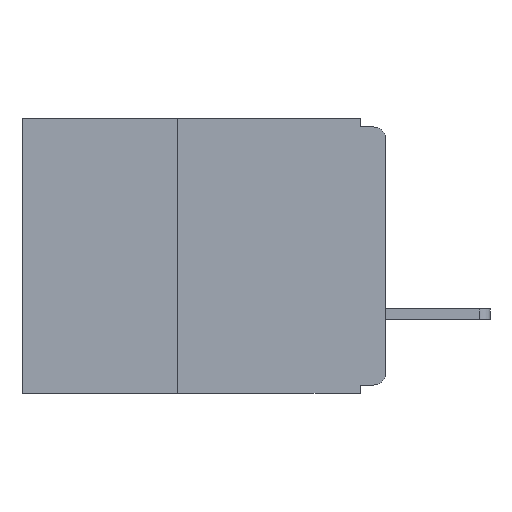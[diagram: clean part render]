
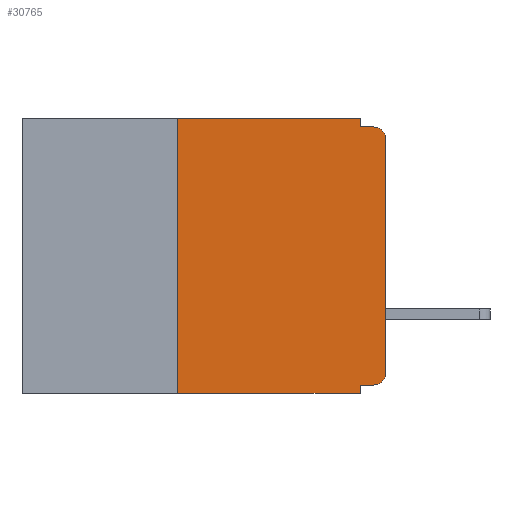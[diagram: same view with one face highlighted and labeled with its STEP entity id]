
A CAD part, left-side view. The second image highlights one B-rep face of the part: STEP entity #30765.
In plain terms, the highlighted planar face has unit normal (-1, 0, 0).
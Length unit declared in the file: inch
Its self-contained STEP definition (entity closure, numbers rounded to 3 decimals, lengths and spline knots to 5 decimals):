
#127 = ORIENTED_EDGE ( 'NONE', *, *, #270, .T. ) ;
#175 = EDGE_CURVE ( 'NONE', #3775, #14281, #20078, .T. ) ;
#227 = EDGE_CURVE ( 'NONE', #13502, #5684, #2865, .T. ) ;
#270 = EDGE_CURVE ( 'NONE', #13502, #5543, #15963, .T. ) ;
#341 = CARTESIAN_POINT ( 'NONE',  ( 0., 0.015, -0.305 ) ) ;
#1022 = CARTESIAN_POINT ( 'NONE',  ( 0., 0.031, -0.33 ) ) ;
#1690 = CARTESIAN_POINT ( 'NONE',  ( 0., 0., -0.32 ) ) ;
#2069 = CARTESIAN_POINT ( 'NONE',  ( 0., 0., 0. ) ) ;
#2689 = CARTESIAN_POINT ( 'NONE',  ( 0., 0., -0.025 ) ) ;
#2794 = CARTESIAN_POINT ( 'NONE',  ( 0., 0.015, -0.32 ) ) ;
#2865 = LINE ( 'NONE', #22515, #29962 ) ;
#2972 = DIRECTION ( 'NONE',  ( 0., 0., -1. ) ) ;
#3122 = ORIENTED_EDGE ( 'NONE', *, *, #25680, .T. ) ;
#3360 = CARTESIAN_POINT ( 'NONE',  ( 0., 0.25, -0.33 ) ) ;
#3447 = AXIS2_PLACEMENT_3D ( 'NONE', #341, #18685, #2972 ) ;
#3775 = VERTEX_POINT ( 'NONE', #32200 ) ;
#4452 = CIRCLE ( 'NONE', #16039, 0.015 ) ;
#5268 = DIRECTION ( 'NONE',  ( 0., -1., 0. ) ) ;
#5543 = VERTEX_POINT ( 'NONE', #8199 ) ;
#5684 = VERTEX_POINT ( 'NONE', #19339 ) ;
#6016 = AXIS2_PLACEMENT_3D ( 'NONE', #25870, #7611, #25985 ) ;
#6354 = DIRECTION ( 'NONE',  ( 0., 0., -1. ) ) ;
#7611 = DIRECTION ( 'NONE',  ( 1., 0., 0. ) ) ;
#7629 = LINE ( 'NONE', #20999, #26948 ) ;
#8135 = CARTESIAN_POINT ( 'NONE',  ( 0., 0., -0.01 ) ) ;
#8155 = CARTESIAN_POINT ( 'NONE',  ( 0., 0.015, -0.025 ) ) ;
#8199 = CARTESIAN_POINT ( 'NONE',  ( 0., 0.031, -0.33 ) ) ;
#8283 = ORIENTED_EDGE ( 'NONE', *, *, #30093, .F. ) ;
#8722 = ORIENTED_EDGE ( 'NONE', *, *, #16659, .F. ) ;
#9437 = ORIENTED_EDGE ( 'NONE', *, *, #17554, .F. ) ;
#9667 = VECTOR ( 'NONE', #30607, 39.37008 ) ;
#10758 = DIRECTION ( 'NONE',  ( 0., 0., -1. ) ) ;
#11637 = FACE_OUTER_BOUND ( 'NONE', #14182, .T. ) ;
#13502 = VERTEX_POINT ( 'NONE', #3360 ) ;
#14021 = CIRCLE ( 'NONE', #3447, 0.015 ) ;
#14182 = EDGE_LOOP ( 'NONE', ( #19670, #3122, #9437, #26862, #8283, #20357, #127, #31648, #8722, #22837 ) ) ;
#14281 = VERTEX_POINT ( 'NONE', #30339 ) ;
#14502 = CARTESIAN_POINT ( 'NONE',  ( 0., 0.437, -0.33 ) ) ;
#14557 = LINE ( 'NONE', #2069, #20733 ) ;
#14693 = CARTESIAN_POINT ( 'NONE',  ( 0., 0.031, -0.32 ) ) ;
#15133 = VECTOR ( 'NONE', #32980, 39.37008 ) ;
#15455 = CARTESIAN_POINT ( 'NONE',  ( 0., 0., -0.305 ) ) ;
#15963 = LINE ( 'NONE', #14502, #15133 ) ;
#16039 = AXIS2_PLACEMENT_3D ( 'NONE', #8155, #26539, #10758 ) ;
#16659 = EDGE_CURVE ( 'NONE', #19332, #19085, #18342, .T. ) ;
#17116 = VECTOR ( 'NONE', #19356, 39.37008 ) ;
#17554 = EDGE_CURVE ( 'NONE', #14281, #29643, #23903, .T. ) ;
#17752 = DIRECTION ( 'NONE',  ( 0., 0., 1. ) ) ;
#18059 = PLANE ( 'NONE',  #6016 ) ;
#18083 = VERTEX_POINT ( 'NONE', #15455 ) ;
#18342 = LINE ( 'NONE', #1690, #9667 ) ;
#18456 = VECTOR ( 'NONE', #6354, 39.37008 ) ;
#18685 = DIRECTION ( 'NONE',  ( -1., 0., 0. ) ) ;
#18797 = LINE ( 'NONE', #1022, #17116 ) ;
#19085 = VERTEX_POINT ( 'NONE', #14693 ) ;
#19332 = VERTEX_POINT ( 'NONE', #2794 ) ;
#19339 = CARTESIAN_POINT ( 'NONE',  ( 0., 0.25, 0. ) ) ;
#19356 = DIRECTION ( 'NONE',  ( 0., 0., -1. ) ) ;
#19670 = ORIENTED_EDGE ( 'NONE', *, *, #30486, .T. ) ;
#20078 = LINE ( 'NONE', #26857, #18456 ) ;
#20357 = ORIENTED_EDGE ( 'NONE', *, *, #227, .F. ) ;
#20733 = VECTOR ( 'NONE', #17752, 39.37008 ) ;
#20999 = CARTESIAN_POINT ( 'NONE',  ( 0., 0.437, 0. ) ) ;
#21227 = DIRECTION ( 'NONE',  ( 0., -1., 0. ) ) ;
#22515 = CARTESIAN_POINT ( 'NONE',  ( 0., 0.25, -0.33 ) ) ;
#22837 = ORIENTED_EDGE ( 'NONE', *, *, #32057, .T. ) ;
#22881 = DIRECTION ( 'NONE',  ( 0., 0., 1. ) ) ;
#23903 = LINE ( 'NONE', #8135, #30097 ) ;
#25680 = EDGE_CURVE ( 'NONE', #27510, #29643, #4452, .T. ) ;
#25870 = CARTESIAN_POINT ( 'NONE',  ( 0., 0.437, 0. ) ) ;
#25985 = DIRECTION ( 'NONE',  ( 0., 0., -1. ) ) ;
#26539 = DIRECTION ( 'NONE',  ( -1., 0., 0. ) ) ;
#26857 = CARTESIAN_POINT ( 'NONE',  ( 0., 0.031, 0. ) ) ;
#26862 = ORIENTED_EDGE ( 'NONE', *, *, #175, .F. ) ;
#26948 = VECTOR ( 'NONE', #5268, 39.37008 ) ;
#27510 = VERTEX_POINT ( 'NONE', #2689 ) ;
#29147 = EDGE_CURVE ( 'NONE', #19085, #5543, #18797, .T. ) ;
#29447 = CARTESIAN_POINT ( 'NONE',  ( 0., 0.015, -0.01 ) ) ;
#29643 = VERTEX_POINT ( 'NONE', #29447 ) ;
#29962 = VECTOR ( 'NONE', #22881, 39.37008 ) ;
#30093 = EDGE_CURVE ( 'NONE', #5684, #3775, #7629, .T. ) ;
#30097 = VECTOR ( 'NONE', #21227, 39.37008 ) ;
#30339 = CARTESIAN_POINT ( 'NONE',  ( 0., 0.031, -0.01 ) ) ;
#30486 = EDGE_CURVE ( 'NONE', #18083, #27510, #14557, .T. ) ;
#30607 = DIRECTION ( 'NONE',  ( 0., 1., 0. ) ) ;
#30765 = ADVANCED_FACE ( 'NONE', ( #11637 ), #18059, .F. ) ;
#31648 = ORIENTED_EDGE ( 'NONE', *, *, #29147, .F. ) ;
#32057 = EDGE_CURVE ( 'NONE', #19332, #18083, #14021, .T. ) ;
#32200 = CARTESIAN_POINT ( 'NONE',  ( 0., 0.031, 0. ) ) ;
#32980 = DIRECTION ( 'NONE',  ( 0., -1., 0. ) ) ;
